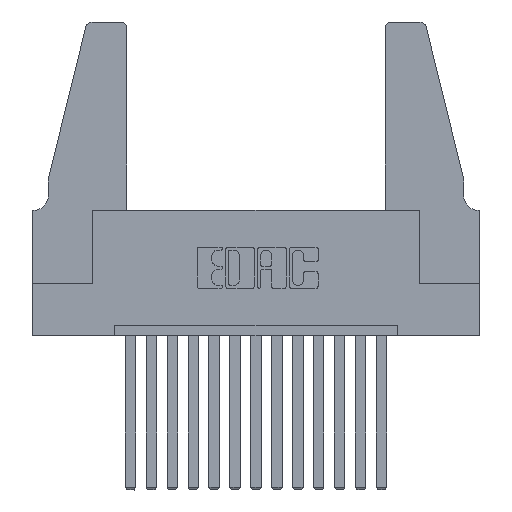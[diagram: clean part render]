
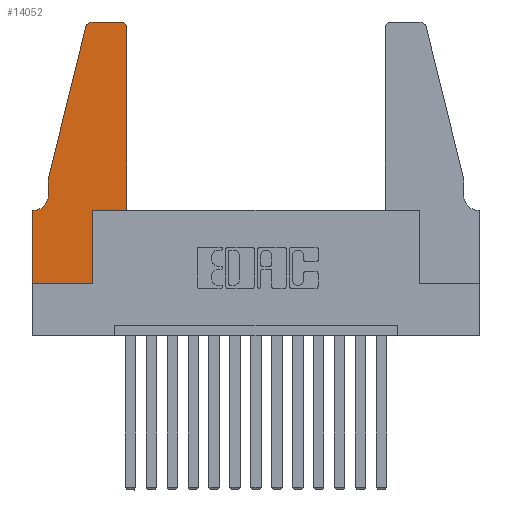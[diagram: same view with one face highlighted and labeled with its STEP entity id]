
A CAD part, top view. The second image highlights one B-rep face of the part: STEP entity #14052.
In plain terms, the highlighted planar face has unit normal (0, 0, 1).
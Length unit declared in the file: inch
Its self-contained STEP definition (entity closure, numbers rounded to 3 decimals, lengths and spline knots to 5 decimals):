
#47 = ORIENTED_EDGE ( 'NONE', *, *, #2740, .T. ) ;
#248 = EDGE_CURVE ( 'NONE', #11338, #1636, #10991, .T. ) ;
#724 = AXIS2_PLACEMENT_3D ( 'NONE', #5720, #3130, #14076 ) ;
#742 = EDGE_CURVE ( 'NONE', #14071, #11338, #5303, .T. ) ;
#857 = CARTESIAN_POINT ( 'NONE',  ( 0.2865, 0.35, 0.37 ) ) ;
#969 = CARTESIAN_POINT ( 'NONE',  ( 0., 0.35, 0.37 ) ) ;
#1326 = DIRECTION ( 'NONE',  ( 1., 0., 0. ) ) ;
#1330 = EDGE_CURVE ( 'NONE', #1636, #6833, #6044, .T. ) ;
#1416 = LINE ( 'NONE', #5382, #2962 ) ;
#1426 = CARTESIAN_POINT ( 'NONE',  ( 0.4505, 1.22, 0.37 ) ) ;
#1562 = VERTEX_POINT ( 'NONE', #1426 ) ;
#1625 = CARTESIAN_POINT ( 'NONE',  ( 0.4205, 1.25, 0.37 ) ) ;
#1636 = VERTEX_POINT ( 'NONE', #6972 ) ;
#1694 = VERTEX_POINT ( 'NONE', #2573 ) ;
#1740 = VERTEX_POINT ( 'NONE', #10250 ) ;
#1821 = VERTEX_POINT ( 'NONE', #969 ) ;
#2092 = EDGE_CURVE ( 'NONE', #2844, #1562, #14148, .T. ) ;
#2556 = LINE ( 'NONE', #13101, #15220 ) ;
#2573 = CARTESIAN_POINT ( 'NONE',  ( 0.2865, 0., 0.37 ) ) ;
#2740 = EDGE_CURVE ( 'NONE', #1694, #11613, #3518, .T. ) ;
#2766 = CARTESIAN_POINT ( 'NONE',  ( 0.0755, 0.5, 0.37 ) ) ;
#2833 = VECTOR ( 'NONE', #5417, 39.37008 ) ;
#2844 = VERTEX_POINT ( 'NONE', #3583 ) ;
#2869 = ORIENTED_EDGE ( 'NONE', *, *, #10325, .T. ) ;
#2962 = VECTOR ( 'NONE', #6679, 39.37008 ) ;
#3115 = VECTOR ( 'NONE', #5311, 39.37008 ) ;
#3130 = DIRECTION ( 'NONE',  ( 0., 0., 1. ) ) ;
#3305 = CARTESIAN_POINT ( 'NONE',  ( 0., 0.35, 0.37 ) ) ;
#3347 = ORIENTED_EDGE ( 'NONE', *, *, #14325, .T. ) ;
#3518 = LINE ( 'NONE', #857, #5420 ) ;
#3583 = CARTESIAN_POINT ( 'NONE',  ( 0.4505, 0.35, 0.37 ) ) ;
#3785 = DIRECTION ( 'NONE',  ( -1., 0., 0. ) ) ;
#3843 = CARTESIAN_POINT ( 'NONE',  ( 0.0055, 0.35, 0.37 ) ) ;
#3962 = ORIENTED_EDGE ( 'NONE', *, *, #12592, .T. ) ;
#4247 = VECTOR ( 'NONE', #8553, 39.37008 ) ;
#4400 = DIRECTION ( 'NONE',  ( 0., 1., 0. ) ) ;
#4688 = VECTOR ( 'NONE', #10657, 39.37008 ) ;
#4715 = ORIENTED_EDGE ( 'NONE', *, *, #13066, .T. ) ;
#5098 = CARTESIAN_POINT ( 'NONE',  ( 0.2605, 1.25, 0.37 ) ) ;
#5103 = CARTESIAN_POINT ( 'NONE',  ( 0.0055, 0.42, 0.37 ) ) ;
#5252 = ORIENTED_EDGE ( 'NONE', *, *, #742, .T. ) ;
#5303 = CIRCLE ( 'NONE', #8226, 0.03 ) ;
#5311 = DIRECTION ( 'NONE',  ( 1., 0., 0. ) ) ;
#5382 = CARTESIAN_POINT ( 'NONE',  ( 0., 0., 0.37 ) ) ;
#5417 = DIRECTION ( 'NONE',  ( 0., -1., 0. ) ) ;
#5420 = VECTOR ( 'NONE', #4400, 39.37008 ) ;
#5506 = VERTEX_POINT ( 'NONE', #1625 ) ;
#5687 = DIRECTION ( 'NONE',  ( 1., 0., 0. ) ) ;
#5720 = CARTESIAN_POINT ( 'NONE',  ( 0.4205, 1.22, 0.37 ) ) ;
#5865 = ORIENTED_EDGE ( 'NONE', *, *, #1330, .T. ) ;
#6044 = LINE ( 'NONE', #12645, #2833 ) ;
#6145 = DIRECTION ( 'NONE',  ( 0., 0., 1. ) ) ;
#6679 = DIRECTION ( 'NONE',  ( 0., -1., 0. ) ) ;
#6833 = VERTEX_POINT ( 'NONE', #9417 ) ;
#6904 = FACE_OUTER_BOUND ( 'NONE', #15480, .T. ) ;
#6972 = CARTESIAN_POINT ( 'NONE',  ( 0.0755, 0.5, 0.37 ) ) ;
#7095 = CARTESIAN_POINT ( 'NONE',  ( 0.4505, 0.35, 0.37 ) ) ;
#7128 = LINE ( 'NONE', #11192, #7883 ) ;
#7421 = CARTESIAN_POINT ( 'NONE',  ( 0.284, 1.22, 0.37 ) ) ;
#7608 = CIRCLE ( 'NONE', #10384, 0.07 ) ;
#7669 = DIRECTION ( 'NONE',  ( 1., 0., 0. ) ) ;
#7754 = AXIS2_PLACEMENT_3D ( 'NONE', #3305, #14260, #5687 ) ;
#7883 = VECTOR ( 'NONE', #7669, 39.37008 ) ;
#8226 = AXIS2_PLACEMENT_3D ( 'NONE', #7421, #6145, #1326 ) ;
#8399 = ORIENTED_EDGE ( 'NONE', *, *, #13825, .T. ) ;
#8553 = DIRECTION ( 'NONE',  ( -1., 0., 0. ) ) ;
#8677 = CARTESIAN_POINT ( 'NONE',  ( 0.25487, 1.22718, 0.37 ) ) ;
#8707 = ORIENTED_EDGE ( 'NONE', *, *, #15445, .T. ) ;
#9417 = CARTESIAN_POINT ( 'NONE',  ( 0.0755, 0.42, 0.37 ) ) ;
#9843 = DIRECTION ( 'NONE',  ( 0., 0., -1. ) ) ;
#10250 = CARTESIAN_POINT ( 'NONE',  ( 0., 0., 0.37 ) ) ;
#10325 = EDGE_CURVE ( 'NONE', #1821, #1740, #1416, .T. ) ;
#10331 = CIRCLE ( 'NONE', #724, 0.03 ) ;
#10384 = AXIS2_PLACEMENT_3D ( 'NONE', #5103, #9843, #3785 ) ;
#10489 = CARTESIAN_POINT ( 'NONE',  ( 0.2865, 0.35, 0.37 ) ) ;
#10657 = DIRECTION ( 'NONE',  ( 0., 1., 0. ) ) ;
#10991 = LINE ( 'NONE', #2766, #13454 ) ;
#11018 = EDGE_CURVE ( 'NONE', #5506, #14071, #13128, .T. ) ;
#11192 = CARTESIAN_POINT ( 'NONE',  ( 0., 0., 0.37 ) ) ;
#11324 = CARTESIAN_POINT ( 'NONE',  ( 0.4505, 0.35, 0.37 ) ) ;
#11338 = VERTEX_POINT ( 'NONE', #8677 ) ;
#11613 = VERTEX_POINT ( 'NONE', #10489 ) ;
#12453 = ORIENTED_EDGE ( 'NONE', *, *, #11018, .T. ) ;
#12592 = EDGE_CURVE ( 'NONE', #1562, #5506, #10331, .T. ) ;
#12645 = CARTESIAN_POINT ( 'NONE',  ( 0.0755, 0.5, 0.37 ) ) ;
#12859 = ORIENTED_EDGE ( 'NONE', *, *, #2092, .T. ) ;
#13017 = CARTESIAN_POINT ( 'NONE',  ( 0.284, 1.25, 0.37 ) ) ;
#13066 = EDGE_CURVE ( 'NONE', #1740, #1694, #7128, .T. ) ;
#13101 = CARTESIAN_POINT ( 'NONE',  ( 0.0755, 0.35, 0.37 ) ) ;
#13128 = LINE ( 'NONE', #5098, #4247 ) ;
#13133 = LINE ( 'NONE', #11324, #3115 ) ;
#13418 = VERTEX_POINT ( 'NONE', #3843 ) ;
#13427 = DIRECTION ( 'NONE',  ( -1., 0., 0. ) ) ;
#13444 = DIRECTION ( 'NONE',  ( -0.239, -0.971, 0. ) ) ;
#13454 = VECTOR ( 'NONE', #13444, 39.37008 ) ;
#13825 = EDGE_CURVE ( 'NONE', #11613, #2844, #13133, .T. ) ;
#14052 = ADVANCED_FACE ( 'NONE', ( #6904 ), #15384, .T. ) ;
#14071 = VERTEX_POINT ( 'NONE', #13017 ) ;
#14076 = DIRECTION ( 'NONE',  ( 1., 0., 0. ) ) ;
#14148 = LINE ( 'NONE', #7095, #4688 ) ;
#14260 = DIRECTION ( 'NONE',  ( 0., 0., 1. ) ) ;
#14325 = EDGE_CURVE ( 'NONE', #13418, #1821, #2556, .T. ) ;
#14911 = ORIENTED_EDGE ( 'NONE', *, *, #248, .T. ) ;
#15220 = VECTOR ( 'NONE', #13427, 39.37008 ) ;
#15384 = PLANE ( 'NONE',  #7754 ) ;
#15445 = EDGE_CURVE ( 'NONE', #6833, #13418, #7608, .T. ) ;
#15480 = EDGE_LOOP ( 'NONE', ( #12453, #5252, #14911, #5865, #8707, #3347, #2869, #4715, #47, #8399, #12859, #3962 ) ) ;
